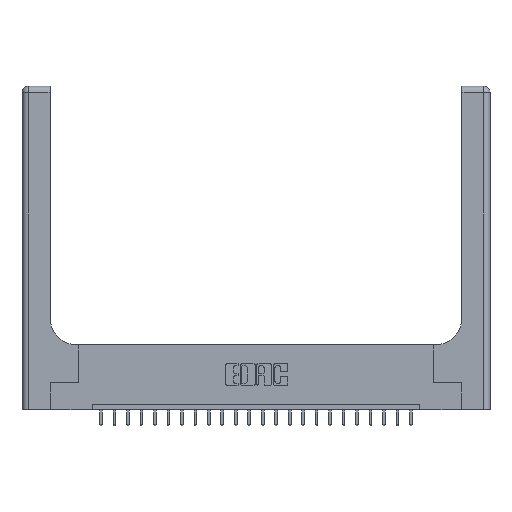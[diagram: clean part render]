
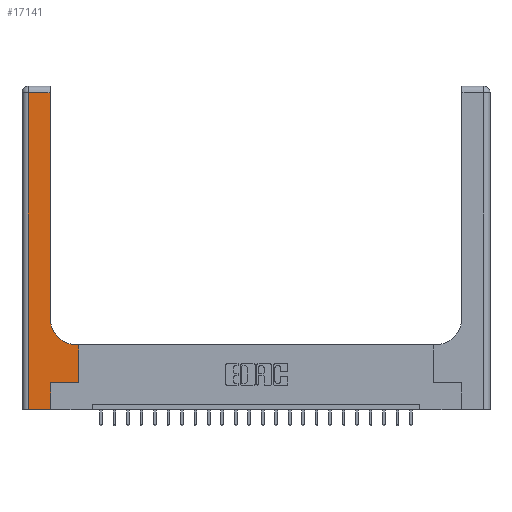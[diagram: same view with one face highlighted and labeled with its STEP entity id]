
A CAD part, top view. The second image highlights one B-rep face of the part: STEP entity #17141.
In plain terms, the highlighted planar face has unit normal (0, 0, 1).
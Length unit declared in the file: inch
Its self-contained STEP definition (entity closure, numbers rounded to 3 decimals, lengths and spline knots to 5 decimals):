
#258 = ORIENTED_EDGE ( 'NONE', *, *, #15145, .T. ) ;
#751 = EDGE_CURVE ( 'NONE', #769, #9579, #8509, .T. ) ;
#769 = VERTEX_POINT ( 'NONE', #10267 ) ;
#1224 = EDGE_LOOP ( 'NONE', ( #7716, #18255, #2411, #7813, #258, #8898, #10057, #2849, #5496 ) ) ;
#1275 = DIRECTION ( 'NONE',  ( -1., 0., 0. ) ) ;
#1352 = VERTEX_POINT ( 'NONE', #20718 ) ;
#1945 = VERTEX_POINT ( 'NONE', #4203 ) ;
#1993 = AXIS2_PLACEMENT_3D ( 'NONE', #8077, #17640, #5949 ) ;
#2031 = PLANE ( 'NONE',  #1993 ) ;
#2411 = ORIENTED_EDGE ( 'NONE', *, *, #4121, .T. ) ;
#2849 = ORIENTED_EDGE ( 'NONE', *, *, #20056, .T. ) ;
#2909 = LINE ( 'NONE', #6616, #7483 ) ;
#3450 = DIRECTION ( 'NONE',  ( -1., 0., 0. ) ) ;
#3708 = CARTESIAN_POINT ( 'NONE',  ( 0.528, 0.25, 0.37 ) ) ;
#4052 = VECTOR ( 'NONE', #18581, 39.37008 ) ;
#4121 = EDGE_CURVE ( 'NONE', #9579, #1945, #19862, .T. ) ;
#4203 = CARTESIAN_POINT ( 'NONE',  ( 0.06, 0., 0.37 ) ) ;
#5252 = DIRECTION ( 'NONE',  ( 0., 0., -1. ) ) ;
#5496 = ORIENTED_EDGE ( 'NONE', *, *, #17632, .T. ) ;
#5683 = CIRCLE ( 'NONE', #14634, 0.25 ) ;
#5855 = DIRECTION ( 'NONE',  ( 0., -1., 0. ) ) ;
#5938 = CARTESIAN_POINT ( 'NONE',  ( 0.06, 3., 0.37 ) ) ;
#5949 = DIRECTION ( 'NONE',  ( -1., 0., 0. ) ) ;
#5963 = CARTESIAN_POINT ( 'NONE',  ( 0.26, 0.85, 0.37 ) ) ;
#6135 = CARTESIAN_POINT ( 'NONE',  ( 0.265, 0.25, 0.37 ) ) ;
#6616 = CARTESIAN_POINT ( 'NONE',  ( 0., 0., 0.37 ) ) ;
#7483 = VECTOR ( 'NONE', #18704, 39.37008 ) ;
#7716 = ORIENTED_EDGE ( 'NONE', *, *, #21255, .T. ) ;
#7813 = ORIENTED_EDGE ( 'NONE', *, *, #19343, .T. ) ;
#7843 = DIRECTION ( 'NONE',  ( 1., 0., 0. ) ) ;
#7987 = CARTESIAN_POINT ( 'NONE',  ( 0.26, 3., 0.37 ) ) ;
#8077 = CARTESIAN_POINT ( 'NONE',  ( 0., 3., 0.37 ) ) ;
#8509 = LINE ( 'NONE', #18920, #17507 ) ;
#8757 = LINE ( 'NONE', #16807, #19399 ) ;
#8898 = ORIENTED_EDGE ( 'NONE', *, *, #21148, .T. ) ;
#9100 = VECTOR ( 'NONE', #1275, 39.37008 ) ;
#9579 = VERTEX_POINT ( 'NONE', #16298 ) ;
#9963 = VERTEX_POINT ( 'NONE', #19037 ) ;
#10015 = VECTOR ( 'NONE', #5855, 39.37008 ) ;
#10057 = ORIENTED_EDGE ( 'NONE', *, *, #21665, .T. ) ;
#10267 = CARTESIAN_POINT ( 'NONE',  ( 0.26, 2.94, 0.37 ) ) ;
#10304 = VERTEX_POINT ( 'NONE', #5963 ) ;
#11364 = CARTESIAN_POINT ( 'NONE',  ( 0.528, 0.6, 0.37 ) ) ;
#11796 = CARTESIAN_POINT ( 'NONE',  ( 0.26, 0.6, 0.37 ) ) ;
#12110 = VERTEX_POINT ( 'NONE', #11364 ) ;
#12319 = DIRECTION ( 'NONE',  ( 1., 0., 0. ) ) ;
#13011 = VERTEX_POINT ( 'NONE', #15255 ) ;
#13798 = LINE ( 'NONE', #7987, #4052 ) ;
#14344 = VECTOR ( 'NONE', #7843, 39.37008 ) ;
#14634 = AXIS2_PLACEMENT_3D ( 'NONE', #21008, #5252, #12319 ) ;
#15127 = DIRECTION ( 'NONE',  ( 0., 1., 0. ) ) ;
#15145 = EDGE_CURVE ( 'NONE', #13011, #1352, #8757, .T. ) ;
#15255 = CARTESIAN_POINT ( 'NONE',  ( 0.265, 0., 0.37 ) ) ;
#16190 = DIRECTION ( 'NONE',  ( 0., 1., 0. ) ) ;
#16278 = FACE_OUTER_BOUND ( 'NONE', #1224, .T. ) ;
#16298 = CARTESIAN_POINT ( 'NONE',  ( 0.06, 2.94, 0.37 ) ) ;
#16723 = LINE ( 'NONE', #11796, #9100 ) ;
#16807 = CARTESIAN_POINT ( 'NONE',  ( 0.265, 0., 0.37 ) ) ;
#17141 = ADVANCED_FACE ( 'NONE', ( #16278 ), #2031, .F. ) ;
#17507 = VECTOR ( 'NONE', #3450, 39.37008 ) ;
#17632 = EDGE_CURVE ( 'NONE', #9963, #10304, #5683, .T. ) ;
#17640 = DIRECTION ( 'NONE',  ( 0., 0., -1. ) ) ;
#18151 = LINE ( 'NONE', #19635, #21154 ) ;
#18255 = ORIENTED_EDGE ( 'NONE', *, *, #751, .T. ) ;
#18581 = DIRECTION ( 'NONE',  ( 0., 1., 0. ) ) ;
#18704 = DIRECTION ( 'NONE',  ( 1., 0., 0. ) ) ;
#18920 = CARTESIAN_POINT ( 'NONE',  ( 0., 2.94, 0.37 ) ) ;
#18935 = VERTEX_POINT ( 'NONE', #3708 ) ;
#19037 = CARTESIAN_POINT ( 'NONE',  ( 0.51, 0.6, 0.37 ) ) ;
#19343 = EDGE_CURVE ( 'NONE', #1945, #13011, #2909, .T. ) ;
#19399 = VECTOR ( 'NONE', #15127, 39.37008 ) ;
#19635 = CARTESIAN_POINT ( 'NONE',  ( 0.528, 0.25, 0.37 ) ) ;
#19862 = LINE ( 'NONE', #5938, #10015 ) ;
#20056 = EDGE_CURVE ( 'NONE', #12110, #9963, #16723, .T. ) ;
#20718 = CARTESIAN_POINT ( 'NONE',  ( 0.265, 0.25, 0.37 ) ) ;
#21008 = CARTESIAN_POINT ( 'NONE',  ( 0.51, 0.85, 0.37 ) ) ;
#21148 = EDGE_CURVE ( 'NONE', #1352, #18935, #21740, .T. ) ;
#21154 = VECTOR ( 'NONE', #16190, 39.37008 ) ;
#21255 = EDGE_CURVE ( 'NONE', #10304, #769, #13798, .T. ) ;
#21665 = EDGE_CURVE ( 'NONE', #18935, #12110, #18151, .T. ) ;
#21740 = LINE ( 'NONE', #6135, #14344 ) ;
